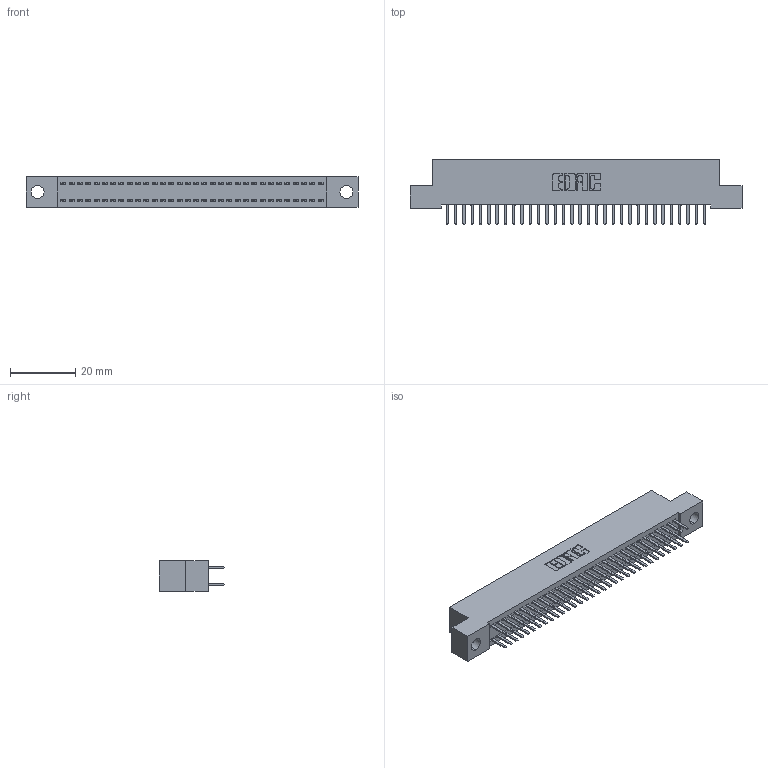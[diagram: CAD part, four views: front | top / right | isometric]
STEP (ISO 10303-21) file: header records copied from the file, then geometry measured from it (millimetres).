
FILE_DESCRIPTION (( 'STEP AP203' ), '1' );
FILE_NAME ('342-064-520-204.STEP', '2018-08-13T07:10:18', ( '' ), ( '' ), 'SwSTEP 2.0', 'SolidWorks 2016', '' );
FILE_SCHEMA (( 'CONFIG_CONTROL_DESIGN' ));
Length unit declared in the file: inch
Products named in the file (3): 342 Part_.156 TH; 345-292-001_345-293-120; 342-064-520-204
Assembly tree (65 placements, depth 2):
  342-064-520-204
    342 Part_.156 TH
    345-292-001_345-293-120  x64
Bounding box: 101.6 x 20.02 x 9.4 mm (x, y, z)
Volume: 8966.3 mm3; surface area: 14106.2 mm2
Topology: 65 solids, 65 shells, 3694 faces, 10731 edges, 6982 vertices
Faces by surface type: plane 2498, cylinder 1196
Entity records: 21865 total; most frequent: CARTESIAN_POINT 3646, ORIENTED_EDGE 3570, DIRECTION 3121, EDGE_CURVE 1785, LINE 1653, VECTOR 1653, VERTEX_POINT 1186, AXIS2_PLACEMENT_3D 734
